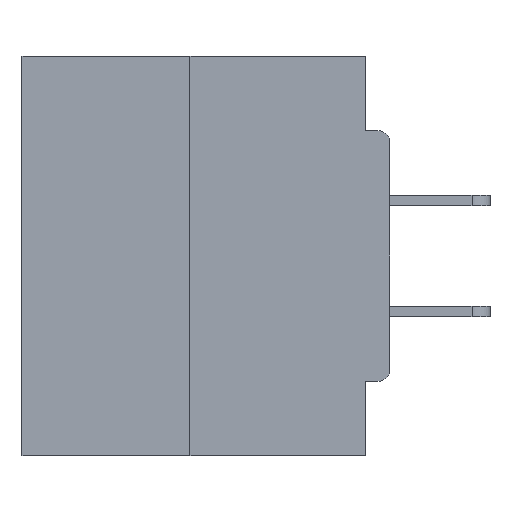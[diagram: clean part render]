
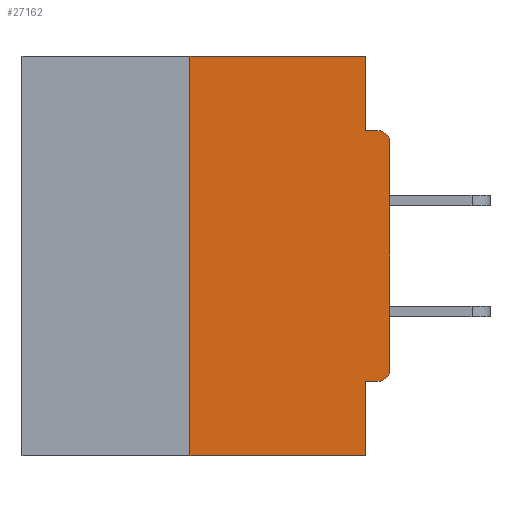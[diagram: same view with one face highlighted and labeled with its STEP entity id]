
A CAD part, left-side view. The second image highlights one B-rep face of the part: STEP entity #27162.
In plain terms, the highlighted planar face has unit normal (-1, 0, 0).
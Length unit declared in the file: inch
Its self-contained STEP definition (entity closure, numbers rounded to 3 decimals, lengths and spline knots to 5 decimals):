
#1983 = VECTOR ( 'NONE', #32811, 39.37008 ) ;
#3061 = EDGE_CURVE ( 'NONE', #43265, #29491, #35876, .T. ) ;
#3082 = VECTOR ( 'NONE', #13477, 39.37008 ) ;
#3151 = LINE ( 'NONE', #37950, #33555 ) ;
#3295 = VECTOR ( 'NONE', #14622, 39.37008 ) ;
#4369 = FACE_OUTER_BOUND ( 'NONE', #13201, .T. ) ;
#7070 = VERTEX_POINT ( 'NONE', #34159 ) ;
#7332 = ORIENTED_EDGE ( 'NONE', *, *, #23946, .F. ) ;
#7431 = AXIS2_PLACEMENT_3D ( 'NONE', #38917, #25718, #35557 ) ;
#8104 = CARTESIAN_POINT ( 'NONE',  ( 0., 0.015, -0.0935 ) ) ;
#8612 = CARTESIAN_POINT ( 'NONE',  ( 0., 0.25, -0.5 ) ) ;
#10397 = VERTEX_POINT ( 'NONE', #30250 ) ;
#10997 = VECTOR ( 'NONE', #25435, 39.37008 ) ;
#11529 = DIRECTION ( 'NONE',  ( -1., 0., 0. ) ) ;
#11719 = EDGE_CURVE ( 'NONE', #30003, #16992, #43144, .T. ) ;
#12074 = EDGE_CURVE ( 'NONE', #12853, #28581, #32047, .T. ) ;
#12075 = LINE ( 'NONE', #35565, #10997 ) ;
#12853 = VERTEX_POINT ( 'NONE', #8612 ) ;
#13201 = EDGE_LOOP ( 'NONE', ( #26327, #38825, #36695, #7332, #31153, #23718, #38838, #21145, #40882, #20626 ) ) ;
#13477 = DIRECTION ( 'NONE',  ( 0., 0., 1. ) ) ;
#14622 = DIRECTION ( 'NONE',  ( 0., -1., 0. ) ) ;
#15691 = EDGE_CURVE ( 'NONE', #10397, #18066, #24558, .T. ) ;
#16276 = EDGE_CURVE ( 'NONE', #28581, #30003, #34486, .T. ) ;
#16965 = DIRECTION ( 'NONE',  ( 0., -1., 0. ) ) ;
#16992 = VERTEX_POINT ( 'NONE', #37732 ) ;
#18066 = VERTEX_POINT ( 'NONE', #19854 ) ;
#19854 = CARTESIAN_POINT ( 'NONE',  ( 0., 0., -0.3915 ) ) ;
#20299 = DIRECTION ( 'NONE',  ( 0., 0., -1. ) ) ;
#20626 = ORIENTED_EDGE ( 'NONE', *, *, #11719, .F. ) ;
#20879 = LINE ( 'NONE', #23400, #3082 ) ;
#21020 = VECTOR ( 'NONE', #26174, 39.37008 ) ;
#21145 = ORIENTED_EDGE ( 'NONE', *, *, #3061, .T. ) ;
#21721 = DIRECTION ( 'NONE',  ( 0., 0., -1. ) ) ;
#22065 = CARTESIAN_POINT ( 'NONE',  ( 0., 0.25, 0. ) ) ;
#22133 = VECTOR ( 'NONE', #16965, 39.37008 ) ;
#23400 = CARTESIAN_POINT ( 'NONE',  ( 0., 0., 0. ) ) ;
#23692 = CARTESIAN_POINT ( 'NONE',  ( 0., 0.031, 0. ) ) ;
#23706 = LINE ( 'NONE', #30594, #22133 ) ;
#23718 = ORIENTED_EDGE ( 'NONE', *, *, #15691, .T. ) ;
#23946 = EDGE_CURVE ( 'NONE', #36643, #7070, #12075, .T. ) ;
#24274 = DIRECTION ( 'NONE',  ( 0., 0., -1. ) ) ;
#24558 = CIRCLE ( 'NONE', #35968, 0.015 ) ;
#25435 = DIRECTION ( 'NONE',  ( 0., 0., -1. ) ) ;
#25718 = DIRECTION ( 'NONE',  ( 1., 0., 0. ) ) ;
#26174 = DIRECTION ( 'NONE',  ( 0., 0., 1. ) ) ;
#26327 = ORIENTED_EDGE ( 'NONE', *, *, #16276, .F. ) ;
#26774 = CARTESIAN_POINT ( 'NONE',  ( 0., 0.015, -0.1085 ) ) ;
#27162 = ADVANCED_FACE ( 'NONE', ( #4369 ), #41587, .F. ) ;
#27221 = DIRECTION ( 'NONE',  ( -1., 0., 0. ) ) ;
#27892 = VECTOR ( 'NONE', #24274, 39.37008 ) ;
#28581 = VERTEX_POINT ( 'NONE', #22065 ) ;
#29491 = VERTEX_POINT ( 'NONE', #8104 ) ;
#30003 = VERTEX_POINT ( 'NONE', #23692 ) ;
#30006 = EDGE_CURVE ( 'NONE', #18066, #43265, #20879, .T. ) ;
#30250 = CARTESIAN_POINT ( 'NONE',  ( 0., 0.015, -0.4065 ) ) ;
#30594 = CARTESIAN_POINT ( 'NONE',  ( 0., 0.46, -0.5 ) ) ;
#31153 = ORIENTED_EDGE ( 'NONE', *, *, #42214, .F. ) ;
#32047 = LINE ( 'NONE', #39645, #21020 ) ;
#32668 = CARTESIAN_POINT ( 'NONE',  ( 0., 0.46, 0. ) ) ;
#32811 = DIRECTION ( 'NONE',  ( 0., -1., 0. ) ) ;
#33268 = CARTESIAN_POINT ( 'NONE',  ( 0., 0., -0.1085 ) ) ;
#33555 = VECTOR ( 'NONE', #37670, 39.37008 ) ;
#33889 = CARTESIAN_POINT ( 'NONE',  ( 0., 0.031, -0.4065 ) ) ;
#34159 = CARTESIAN_POINT ( 'NONE',  ( 0., 0.031, -0.5 ) ) ;
#34410 = CARTESIAN_POINT ( 'NONE',  ( 0., 0.031, 0. ) ) ;
#34486 = LINE ( 'NONE', #32668, #1983 ) ;
#35557 = DIRECTION ( 'NONE',  ( 0., 0., -1. ) ) ;
#35565 = CARTESIAN_POINT ( 'NONE',  ( 0., 0.031, -0.5 ) ) ;
#35876 = CIRCLE ( 'NONE', #39540, 0.015 ) ;
#35968 = AXIS2_PLACEMENT_3D ( 'NONE', #41839, #11529, #21721 ) ;
#35992 = EDGE_CURVE ( 'NONE', #12853, #7070, #23706, .T. ) ;
#36108 = EDGE_CURVE ( 'NONE', #16992, #29491, #40000, .T. ) ;
#36643 = VERTEX_POINT ( 'NONE', #33889 ) ;
#36695 = ORIENTED_EDGE ( 'NONE', *, *, #35992, .T. ) ;
#37670 = DIRECTION ( 'NONE',  ( 0., 1., 0. ) ) ;
#37732 = CARTESIAN_POINT ( 'NONE',  ( 0., 0.031, -0.0935 ) ) ;
#37950 = CARTESIAN_POINT ( 'NONE',  ( 0., 0., -0.4065 ) ) ;
#38825 = ORIENTED_EDGE ( 'NONE', *, *, #12074, .F. ) ;
#38838 = ORIENTED_EDGE ( 'NONE', *, *, #30006, .T. ) ;
#38917 = CARTESIAN_POINT ( 'NONE',  ( 0., 0.46, 0. ) ) ;
#39540 = AXIS2_PLACEMENT_3D ( 'NONE', #26774, #27221, #20299 ) ;
#39645 = CARTESIAN_POINT ( 'NONE',  ( 0., 0.25, 0. ) ) ;
#40000 = LINE ( 'NONE', #41285, #3295 ) ;
#40882 = ORIENTED_EDGE ( 'NONE', *, *, #36108, .F. ) ;
#41285 = CARTESIAN_POINT ( 'NONE',  ( 0., 0., -0.0935 ) ) ;
#41587 = PLANE ( 'NONE',  #7431 ) ;
#41839 = CARTESIAN_POINT ( 'NONE',  ( 0., 0.015, -0.3915 ) ) ;
#42214 = EDGE_CURVE ( 'NONE', #10397, #36643, #3151, .T. ) ;
#43144 = LINE ( 'NONE', #34410, #27892 ) ;
#43265 = VERTEX_POINT ( 'NONE', #33268 ) ;
